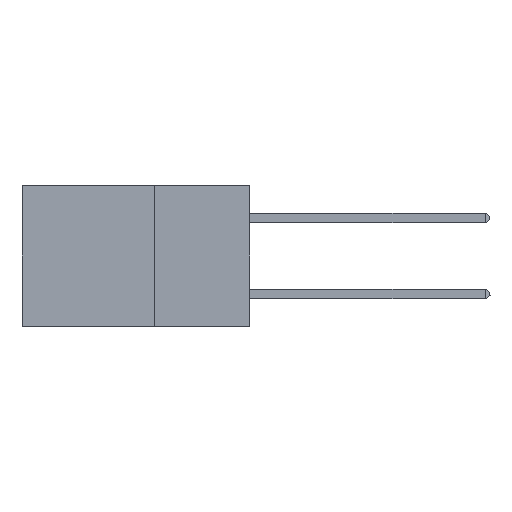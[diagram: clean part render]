
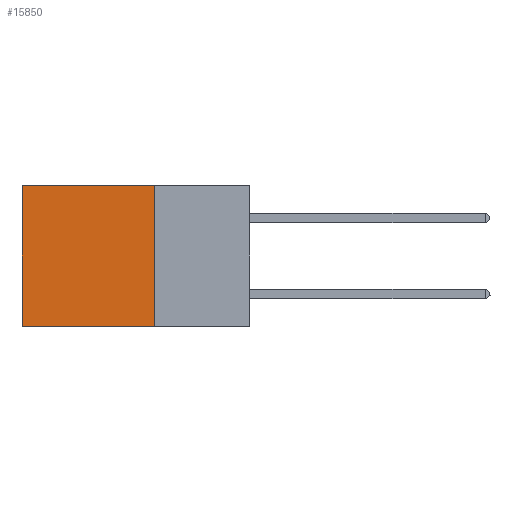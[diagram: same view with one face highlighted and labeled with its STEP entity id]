
A CAD part, left-side view. The second image highlights one B-rep face of the part: STEP entity #15850.
In plain terms, the highlighted planar face has unit normal (-1, 0, 0).
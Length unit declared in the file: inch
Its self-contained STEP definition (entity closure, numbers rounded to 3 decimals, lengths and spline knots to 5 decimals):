
#1901 = VERTEX_POINT ( 'NONE', #12747 ) ;
#2836 = VECTOR ( 'NONE', #4325, 39.37008 ) ;
#2923 = EDGE_CURVE ( 'NONE', #5698, #26180, #26567, .T. ) ;
#3510 = VECTOR ( 'NONE', #5544, 39.37008 ) ;
#4325 = DIRECTION ( 'NONE',  ( 0., 0., -1. ) ) ;
#5544 = DIRECTION ( 'NONE',  ( 0., 0., -1. ) ) ;
#5698 = VERTEX_POINT ( 'NONE', #25888 ) ;
#6426 = CARTESIAN_POINT ( 'NONE',  ( 0.2875, 0.25, 0. ) ) ;
#7146 = LINE ( 'NONE', #13878, #3510 ) ;
#7563 = EDGE_CURVE ( 'NONE', #1901, #5698, #7146, .T. ) ;
#7630 = CARTESIAN_POINT ( 'NONE',  ( 0.2875, 0.25, 0. ) ) ;
#8821 = DIRECTION ( 'NONE',  ( 1., 0., 0. ) ) ;
#10264 = VECTOR ( 'NONE', #22077, 39.37008 ) ;
#11174 = CARTESIAN_POINT ( 'NONE',  ( 0.2875, 0.25, -0.37 ) ) ;
#12036 = LINE ( 'NONE', #18685, #2836 ) ;
#12246 = AXIS2_PLACEMENT_3D ( 'NONE', #6426, #8821, #15024 ) ;
#12747 = CARTESIAN_POINT ( 'NONE',  ( 0.2875, 0.25, 0. ) ) ;
#12773 = ORIENTED_EDGE ( 'NONE', *, *, #2923, .F. ) ;
#12867 = VECTOR ( 'NONE', #15776, 39.37008 ) ;
#12906 = CARTESIAN_POINT ( 'NONE',  ( 0.2875, 0.6, -0.37 ) ) ;
#13878 = CARTESIAN_POINT ( 'NONE',  ( 0.2875, 0.25, 0. ) ) ;
#13904 = EDGE_CURVE ( 'NONE', #14730, #26180, #12036, .T. ) ;
#14730 = VERTEX_POINT ( 'NONE', #20398 ) ;
#14865 = FACE_OUTER_BOUND ( 'NONE', #25897, .T. ) ;
#15024 = DIRECTION ( 'NONE',  ( 0., 0., -1. ) ) ;
#15776 = DIRECTION ( 'NONE',  ( 0., 1., 0. ) ) ;
#15850 = ADVANCED_FACE ( 'NONE', ( #14865 ), #21094, .F. ) ;
#17891 = EDGE_CURVE ( 'NONE', #1901, #14730, #19698, .T. ) ;
#18685 = CARTESIAN_POINT ( 'NONE',  ( 0.2875, 0.6, 0. ) ) ;
#19458 = ORIENTED_EDGE ( 'NONE', *, *, #17891, .T. ) ;
#19698 = LINE ( 'NONE', #7630, #12867 ) ;
#20398 = CARTESIAN_POINT ( 'NONE',  ( 0.2875, 0.6, 0. ) ) ;
#21094 = PLANE ( 'NONE',  #12246 ) ;
#22077 = DIRECTION ( 'NONE',  ( 0., 1., 0. ) ) ;
#22830 = ORIENTED_EDGE ( 'NONE', *, *, #13904, .T. ) ;
#25431 = ORIENTED_EDGE ( 'NONE', *, *, #7563, .F. ) ;
#25888 = CARTESIAN_POINT ( 'NONE',  ( 0.2875, 0.25, -0.37 ) ) ;
#25897 = EDGE_LOOP ( 'NONE', ( #22830, #12773, #25431, #19458 ) ) ;
#26180 = VERTEX_POINT ( 'NONE', #12906 ) ;
#26567 = LINE ( 'NONE', #11174, #10264 ) ;
